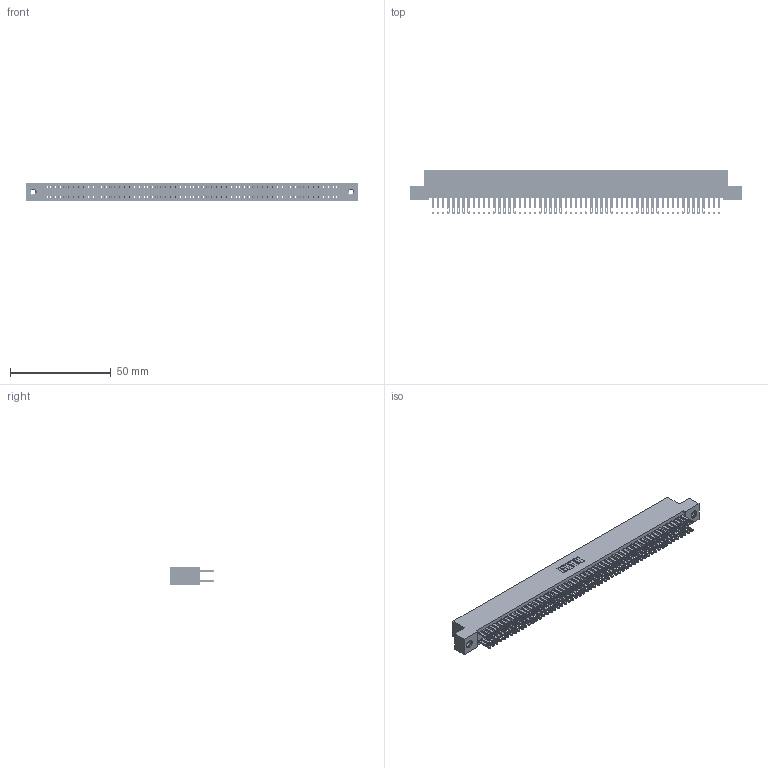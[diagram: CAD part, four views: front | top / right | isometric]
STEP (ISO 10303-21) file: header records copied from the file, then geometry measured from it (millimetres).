
FILE_DESCRIPTION (( 'STEP AP203' ), '1' );
FILE_NAME ('342-114-500-208.STEP', '2019-10-04T21:20:10', ( '' ), ( '' ), 'SwSTEP 2.0', 'SolidWorks 2016', '' );
FILE_SCHEMA (( 'CONFIG_CONTROL_DESIGN' ));
Length unit declared in the file: inch
Products named in the file (4): 342 Part_TI; 345-292-001_345-293-100; 345-250-001_345-250-003-102; 342-114-500-208
Assembly tree (117 placements, depth 2):
  342-114-500-208
    342 Part_TI
    345-292-001_345-293-100  x114
    345-250-001_345-250-003-102  x2
Bounding box: 165.1 x 21.85 x 9.4 mm (x, y, z)
Volume: 15247.9 mm3; surface area: 26291.1 mm2
Topology: 117 solids, 117 shells, 5642 faces, 17193 edges, 11454 vertices
Faces by surface type: plane 3518, cylinder 2108, cone 12, torus 4
Entity records: 35714 total; most frequent: CARTESIAN_POINT 5881, ORIENTED_EDGE 5810, DIRECTION 5031, EDGE_CURVE 2905, LINE 2753, VECTOR 2753, VERTEX_POINT 1932, AXIS2_PLACEMENT_3D 1139
